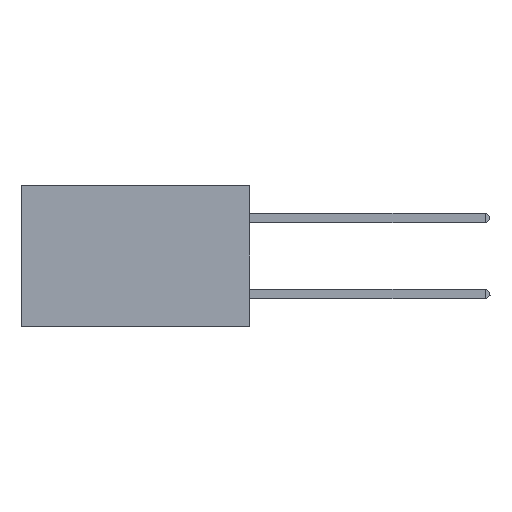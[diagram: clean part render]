
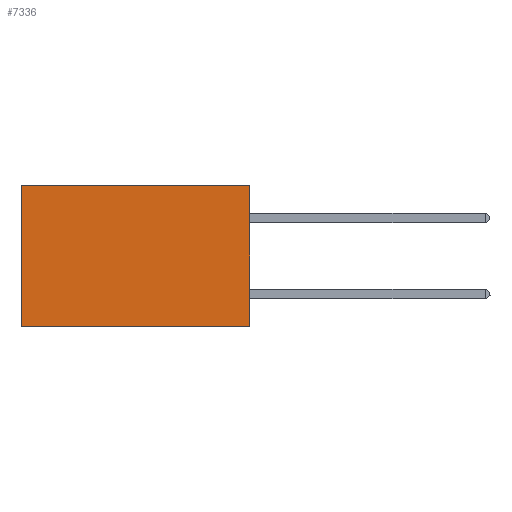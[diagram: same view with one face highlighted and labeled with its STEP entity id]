
A CAD part, left-side view. The second image highlights one B-rep face of the part: STEP entity #7336.
In plain terms, the highlighted planar face has unit normal (-1, 0, 0).
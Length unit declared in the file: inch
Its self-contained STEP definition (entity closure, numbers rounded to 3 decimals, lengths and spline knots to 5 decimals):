
#1577 = FACE_OUTER_BOUND ( 'NONE', #11305, .T. ) ;
#1672 = DIRECTION ( 'NONE',  ( 0., 1., 0. ) ) ;
#2785 = EDGE_CURVE ( 'NONE', #22354, #33492, #30369, .T. ) ;
#3744 = CARTESIAN_POINT ( 'NONE',  ( 0.2875, 0., 0. ) ) ;
#3921 = VECTOR ( 'NONE', #15277, 39.37008 ) ;
#4825 = PLANE ( 'NONE',  #22516 ) ;
#6711 = CARTESIAN_POINT ( 'NONE',  ( 0.2875, 0., 0. ) ) ;
#7336 = ADVANCED_FACE ( 'NONE', ( #1577 ), #4825, .F. ) ;
#9280 = EDGE_CURVE ( 'NONE', #29796, #22354, #32659, .T. ) ;
#11305 = EDGE_LOOP ( 'NONE', ( #17223, #20852, #14703, #32670 ) ) ;
#13910 = CARTESIAN_POINT ( 'NONE',  ( 0.2875, 0.6, 0. ) ) ;
#14703 = ORIENTED_EDGE ( 'NONE', *, *, #9280, .F. ) ;
#15206 = EDGE_CURVE ( 'NONE', #29796, #21776, #38074, .T. ) ;
#15277 = DIRECTION ( 'NONE',  ( 0., 0., -1. ) ) ;
#17223 = ORIENTED_EDGE ( 'NONE', *, *, #36011, .T. ) ;
#18542 = LINE ( 'NONE', #36747, #3921 ) ;
#18870 = CARTESIAN_POINT ( 'NONE',  ( 0.2875, 0., 0. ) ) ;
#19390 = DIRECTION ( 'NONE',  ( 0., 0., -1. ) ) ;
#19730 = CARTESIAN_POINT ( 'NONE',  ( 0.2875, 0., -0.37 ) ) ;
#20852 = ORIENTED_EDGE ( 'NONE', *, *, #2785, .F. ) ;
#21776 = VERTEX_POINT ( 'NONE', #13910 ) ;
#22354 = VERTEX_POINT ( 'NONE', #23498 ) ;
#22516 = AXIS2_PLACEMENT_3D ( 'NONE', #29028, #32077, #29416 ) ;
#22846 = VECTOR ( 'NONE', #31249, 39.37008 ) ;
#23498 = CARTESIAN_POINT ( 'NONE',  ( 0.2875, 0., -0.37 ) ) ;
#27466 = VECTOR ( 'NONE', #1672, 39.37008 ) ;
#29028 = CARTESIAN_POINT ( 'NONE',  ( 0.2875, 0., 0. ) ) ;
#29416 = DIRECTION ( 'NONE',  ( 0., 0., -1. ) ) ;
#29796 = VERTEX_POINT ( 'NONE', #6711 ) ;
#30369 = LINE ( 'NONE', #19730, #27466 ) ;
#31249 = DIRECTION ( 'NONE',  ( 0., 1., 0. ) ) ;
#32077 = DIRECTION ( 'NONE',  ( 1., 0., 0. ) ) ;
#32659 = LINE ( 'NONE', #3744, #37384 ) ;
#32670 = ORIENTED_EDGE ( 'NONE', *, *, #15206, .T. ) ;
#33492 = VERTEX_POINT ( 'NONE', #37095 ) ;
#36011 = EDGE_CURVE ( 'NONE', #21776, #33492, #18542, .T. ) ;
#36747 = CARTESIAN_POINT ( 'NONE',  ( 0.2875, 0.6, 0. ) ) ;
#37095 = CARTESIAN_POINT ( 'NONE',  ( 0.2875, 0.6, -0.37 ) ) ;
#37384 = VECTOR ( 'NONE', #19390, 39.37008 ) ;
#38074 = LINE ( 'NONE', #18870, #22846 ) ;
